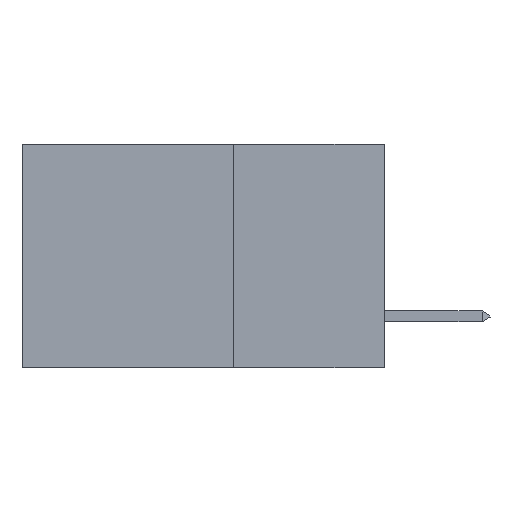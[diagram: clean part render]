
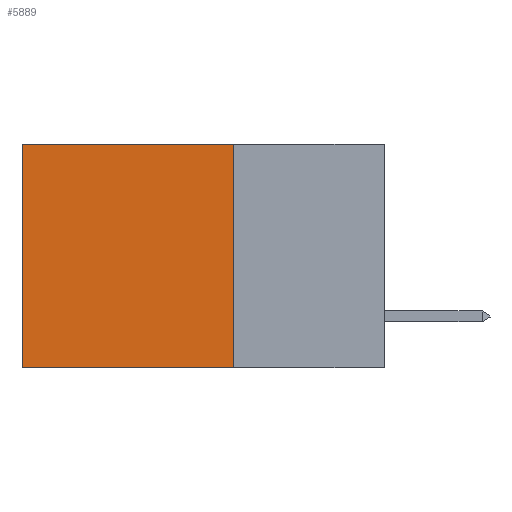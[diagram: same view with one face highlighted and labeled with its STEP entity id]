
A CAD part, left-side view. The second image highlights one B-rep face of the part: STEP entity #5889.
In plain terms, the highlighted planar face has unit normal (-1, 0, 0).
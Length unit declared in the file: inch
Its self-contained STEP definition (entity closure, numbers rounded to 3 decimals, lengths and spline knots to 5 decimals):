
#217 = VECTOR ( 'NONE', #8039, 39.37008 ) ;
#369 = DIRECTION ( 'NONE',  ( 0., 1., 0. ) ) ;
#376 = VERTEX_POINT ( 'NONE', #4739 ) ;
#503 = VERTEX_POINT ( 'NONE', #2325 ) ;
#1045 = ORIENTED_EDGE ( 'NONE', *, *, #7055, .F. ) ;
#1111 = ORIENTED_EDGE ( 'NONE', *, *, #10924, .T. ) ;
#1349 = LINE ( 'NONE', #7305, #2459 ) ;
#1976 = CARTESIAN_POINT ( 'NONE',  ( 0.2875, 0.25, -0.37 ) ) ;
#2325 = CARTESIAN_POINT ( 'NONE',  ( 0.2875, 0.6, -0.37 ) ) ;
#2459 = VECTOR ( 'NONE', #369, 39.37008 ) ;
#3250 = LINE ( 'NONE', #9782, #217 ) ;
#3751 = DIRECTION ( 'NONE',  ( 0., 1., 0. ) ) ;
#3916 = CARTESIAN_POINT ( 'NONE',  ( 0.2875, 0.25, 0. ) ) ;
#4047 = ORIENTED_EDGE ( 'NONE', *, *, #11262, .T. ) ;
#4739 = CARTESIAN_POINT ( 'NONE',  ( 0.2875, 0.6, 0. ) ) ;
#4930 = CARTESIAN_POINT ( 'NONE',  ( 0.2875, 0.25, 0. ) ) ;
#5033 = VERTEX_POINT ( 'NONE', #3916 ) ;
#5548 = EDGE_LOOP ( 'NONE', ( #4047, #10231, #1045, #1111 ) ) ;
#5885 = CARTESIAN_POINT ( 'NONE',  ( 0.2875, 0.25, -0.37 ) ) ;
#5889 = ADVANCED_FACE ( 'NONE', ( #7447 ), #10253, .F. ) ;
#5893 = DIRECTION ( 'NONE',  ( 0., 0., -1. ) ) ;
#7031 = AXIS2_PLACEMENT_3D ( 'NONE', #8434, #11120, #5893 ) ;
#7055 = EDGE_CURVE ( 'NONE', #5033, #7245, #7979, .T. ) ;
#7245 = VERTEX_POINT ( 'NONE', #5885 ) ;
#7305 = CARTESIAN_POINT ( 'NONE',  ( 0.2875, 0.25, 0. ) ) ;
#7447 = FACE_OUTER_BOUND ( 'NONE', #5548, .T. ) ;
#7759 = EDGE_CURVE ( 'NONE', #7245, #503, #9193, .T. ) ;
#7979 = LINE ( 'NONE', #4930, #10872 ) ;
#8039 = DIRECTION ( 'NONE',  ( 0., 0., -1. ) ) ;
#8434 = CARTESIAN_POINT ( 'NONE',  ( 0.2875, 0.25, 0. ) ) ;
#9193 = LINE ( 'NONE', #1976, #10852 ) ;
#9626 = DIRECTION ( 'NONE',  ( 0., 0., -1. ) ) ;
#9782 = CARTESIAN_POINT ( 'NONE',  ( 0.2875, 0.6, 0. ) ) ;
#10231 = ORIENTED_EDGE ( 'NONE', *, *, #7759, .F. ) ;
#10253 = PLANE ( 'NONE',  #7031 ) ;
#10852 = VECTOR ( 'NONE', #3751, 39.37008 ) ;
#10872 = VECTOR ( 'NONE', #9626, 39.37008 ) ;
#10924 = EDGE_CURVE ( 'NONE', #5033, #376, #1349, .T. ) ;
#11120 = DIRECTION ( 'NONE',  ( 1., 0., 0. ) ) ;
#11262 = EDGE_CURVE ( 'NONE', #376, #503, #3250, .T. ) ;
